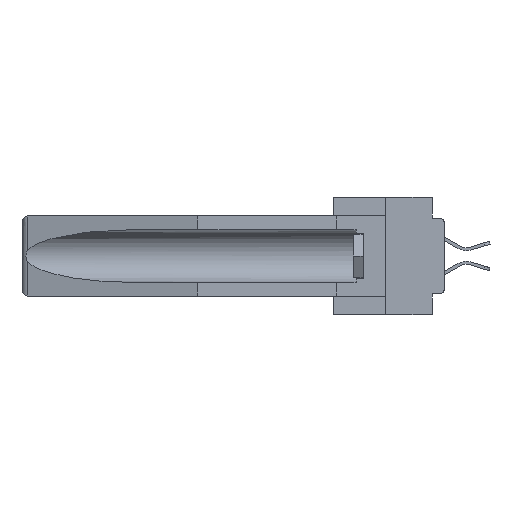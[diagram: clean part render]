
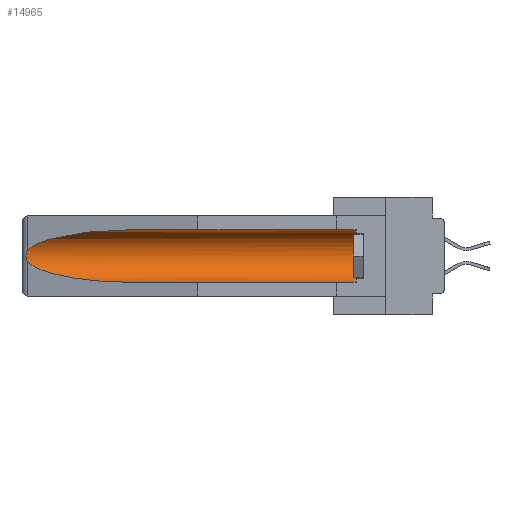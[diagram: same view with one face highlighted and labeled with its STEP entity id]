
A CAD part, left-side view. The second image highlights one B-rep face of the part: STEP entity #14965.
In plain terms, the highlighted cylindrical face has radius 2.857 mm (diameter 5.715 mm), a partial arc.
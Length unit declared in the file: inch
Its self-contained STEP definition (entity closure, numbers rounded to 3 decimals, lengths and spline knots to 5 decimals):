
#629 = CARTESIAN_POINT ( 'NONE',  ( 0.21114, 1.30732, -0.059 ) ) ;
#1026 = CARTESIAN_POINT ( 'NONE',  ( 0.26597, 1.5296, -0.19026 ) ) ;
#1091 = VERTEX_POINT ( 'NONE', #21687 ) ;
#1193 = AXIS2_PLACEMENT_3D ( 'NONE', #34064, #31410, #34187 ) ;
#1606 = EDGE_CURVE ( 'NONE', #7830, #4509, #35229, .T. ) ;
#1672 = ORIENTED_EDGE ( 'NONE', *, *, #32427, .T. ) ;
#1938 = ORIENTED_EDGE ( 'NONE', *, *, #1606, .F. ) ;
#2072 = AXIS2_PLACEMENT_3D ( 'NONE', #14106, #8639, #33305 ) ;
#2261 = DIRECTION ( 'NONE',  ( 0., 1., 0. ) ) ;
#3169 = CARTESIAN_POINT ( 'NONE',  ( 0.26597, 1.52961, -0.15275 ) ) ;
#3642 = CARTESIAN_POINT ( 'NONE',  ( 0.26537, 1.52718, -0.14972 ) ) ;
#4107 = CARTESIAN_POINT ( 'NONE',  ( 0.2675, 1.53308, -0.17534 ) ) ;
#4509 = VERTEX_POINT ( 'NONE', #30976 ) ;
#5463 = CARTESIAN_POINT ( 'NONE',  ( 0.21114, 1.30732, -0.284 ) ) ;
#5758 = CARTESIAN_POINT ( 'NONE',  ( 0.26537, 1.52718, -0.14972 ) ) ;
#6796 = FACE_OUTER_BOUND ( 'NONE', #18599, .T. ) ;
#7768 = EDGE_CURVE ( 'NONE', #1091, #24221, #20537, .T. ) ;
#7830 = VERTEX_POINT ( 'NONE', #9113 ) ;
#8639 = DIRECTION ( 'NONE',  ( 0., 1., 0. ) ) ;
#9113 = CARTESIAN_POINT ( 'NONE',  ( 0.155, 0.126, -0.284 ) ) ;
#9720 = CARTESIAN_POINT ( 'NONE',  ( 0.2673, 1.53269, -0.17917 ) ) ;
#10946 = CARTESIAN_POINT ( 'NONE',  ( 0.26537, 1.52718, -0.19328 ) ) ;
#12473 = CARTESIAN_POINT ( 'NONE',  ( 0.155, 0.126, -0.059 ) ) ;
#12856 = CARTESIAN_POINT ( 'NONE',  ( 0.26537, 1.52718, -0.19328 ) ) ;
#13595 = CYLINDRICAL_SURFACE ( 'NONE', #2072, 0.1125 ) ;
#14060 = DIRECTION ( 'NONE',  ( 0., 1., 0. ) ) ;
#14106 = CARTESIAN_POINT ( 'NONE',  ( 0.155, -0.30754, -0.1715 ) ) ;
#14636 = CIRCLE ( 'NONE', #1193, 0.1125 ) ;
#14847 = CARTESIAN_POINT ( 'NONE',  ( 0.2675, 1.53308, -0.16763 ) ) ;
#14965 = ADVANCED_FACE ( 'NONE', ( #6796 ), #13595, .F. ) ;
#16325 =( BOUNDED_CURVE ( )  B_SPLINE_CURVE ( 3, ( #10946, #21828, #5463, #32890 ),
 .UNSPECIFIED., .F., .F. ) 
 B_SPLINE_CURVE_WITH_KNOTS ( ( 4, 4 ),
 ( 0.1948, 1.5708 ),
 .UNSPECIFIED. ) 
 CURVE ( )  GEOMETRIC_REPRESENTATION_ITEM ( )  RATIONAL_B_SPLINE_CURVE ( ( 1., 0.848, 0.848, 1. ) ) 
 REPRESENTATION_ITEM ( '' )  );
#17043 = CARTESIAN_POINT ( 'NONE',  ( 0.155, -0.30754, -0.284 ) ) ;
#18391 = CARTESIAN_POINT ( 'NONE',  ( 0.26537, 1.52718, -0.19328 ) ) ;
#18599 = EDGE_LOOP ( 'NONE', ( #30736, #31265, #1672, #1938, #34126, #22580 ) ) ;
#18925 = LINE ( 'NONE', #24628, #19373 ) ;
#19373 = VECTOR ( 'NONE', #2261, 39.37008 ) ;
#19374 = CARTESIAN_POINT ( 'NONE',  ( 0.155, 1.07973, -0.059 ) ) ;
#19615 = CARTESIAN_POINT ( 'NONE',  ( 0.155, 1.07973, -0.059 ) ) ;
#20537 = B_SPLINE_CURVE_WITH_KNOTS ( 'NONE', 3,
 ( #3642, #3169, #22661, #33582, #14847, #4107, #9720, #31401, #1026, #12856 ),
 .UNSPECIFIED., .F., .F.,
 ( 4, 2, 2, 2, 4 ),
 ( 0., 0.00029, 0.00058, 0.00087, 0.00117 ),
 .UNSPECIFIED. ) ;
#21687 = CARTESIAN_POINT ( 'NONE',  ( 0.26537, 1.52718, -0.14972 ) ) ;
#21828 = CARTESIAN_POINT ( 'NONE',  ( 0.25451, 1.48313, -0.24835 ) ) ;
#22580 = ORIENTED_EDGE ( 'NONE', *, *, #25965, .T. ) ;
#22661 = CARTESIAN_POINT ( 'NONE',  ( 0.26654, 1.53092, -0.15636 ) ) ;
#22745 =( BOUNDED_CURVE ( )  B_SPLINE_CURVE ( 3, ( #19615, #629, #30537, #5758 ),
 .UNSPECIFIED., .F., .T. ) 
 B_SPLINE_CURVE_WITH_KNOTS ( ( 4, 4 ),
 ( 4.71239, 6.08839 ),
 .UNSPECIFIED. ) 
 CURVE ( )  GEOMETRIC_REPRESENTATION_ITEM ( )  RATIONAL_B_SPLINE_CURVE ( ( 1., 0.848, 0.848, 1. ) ) 
 REPRESENTATION_ITEM ( '' )  );
#23682 = VERTEX_POINT ( 'NONE', #19374 ) ;
#24221 = VERTEX_POINT ( 'NONE', #18391 ) ;
#24628 = CARTESIAN_POINT ( 'NONE',  ( 0.155, -0.30754, -0.059 ) ) ;
#25965 = EDGE_CURVE ( 'NONE', #26340, #23682, #18925, .T. ) ;
#26340 = VERTEX_POINT ( 'NONE', #12473 ) ;
#26391 = EDGE_CURVE ( 'NONE', #7830, #26340, #14636, .T. ) ;
#30419 = EDGE_CURVE ( 'NONE', #23682, #1091, #22745, .T. ) ;
#30537 = CARTESIAN_POINT ( 'NONE',  ( 0.25451, 1.48313, -0.09465 ) ) ;
#30736 = ORIENTED_EDGE ( 'NONE', *, *, #30419, .T. ) ;
#30976 = CARTESIAN_POINT ( 'NONE',  ( 0.155, 1.07973, -0.284 ) ) ;
#31265 = ORIENTED_EDGE ( 'NONE', *, *, #7768, .T. ) ;
#31401 = CARTESIAN_POINT ( 'NONE',  ( 0.26655, 1.53094, -0.18657 ) ) ;
#31410 = DIRECTION ( 'NONE',  ( 0., -1., 0. ) ) ;
#32427 = EDGE_CURVE ( 'NONE', #24221, #4509, #16325, .T. ) ;
#32890 = CARTESIAN_POINT ( 'NONE',  ( 0.155, 1.07973, -0.284 ) ) ;
#33305 = DIRECTION ( 'NONE',  ( 0., 0., 1. ) ) ;
#33582 = CARTESIAN_POINT ( 'NONE',  ( 0.2673, 1.5327, -0.16383 ) ) ;
#34064 = CARTESIAN_POINT ( 'NONE',  ( 0.155, 0.126, -0.1715 ) ) ;
#34126 = ORIENTED_EDGE ( 'NONE', *, *, #26391, .T. ) ;
#34187 = DIRECTION ( 'NONE',  ( 0., 0., 1. ) ) ;
#34821 = VECTOR ( 'NONE', #14060, 39.37008 ) ;
#35229 = LINE ( 'NONE', #17043, #34821 ) ;
